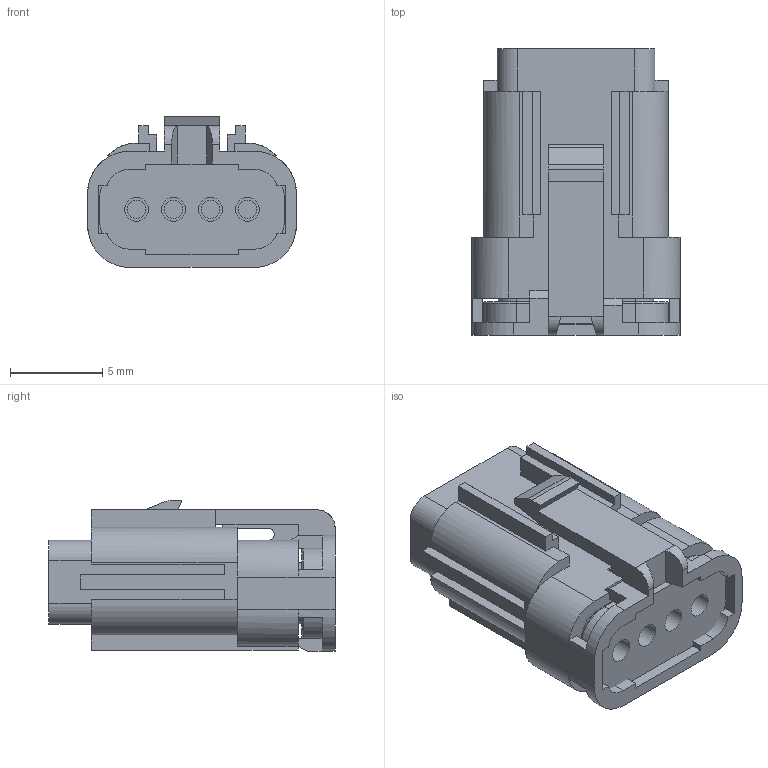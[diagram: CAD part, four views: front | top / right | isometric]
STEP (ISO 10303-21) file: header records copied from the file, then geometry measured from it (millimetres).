
FILE_DESCRIPTION (( 'STEP AP203' ), '1' );
FILE_NAME ('566-004-000-810.STEP', '2021-09-21T19:01:19', ( '' ), ( '' ), 'SwSTEP 2.0', 'SolidWorks 2020', '' );
FILE_SCHEMA (( 'CONFIG_CONTROL_DESIGN' ));
Length unit declared in the file: millimetre
Products named in the file (1): 566-004-000-810
Bounding box: 11.3 x 15.5 x 8.18 mm (x, y, z)
Volume: 747.5 mm3; surface area: 1376.2 mm2
Topology: 2 solids, 2 shells, 462 faces, 1278 edges, 827 vertices
Faces by surface type: plane 355, cylinder 87, torus 16, cone 4
Entity records: 14665 total; most frequent: CARTESIAN_POINT 2574, ORIENTED_EDGE 2556, DIRECTION 2422, EDGE_CURVE 1278, VECTOR 1056, LINE 1056, VERTEX_POINT 827, AXIS2_PLACEMENT_3D 683
